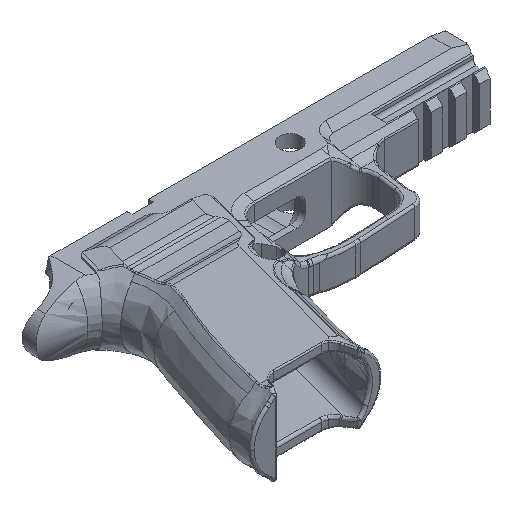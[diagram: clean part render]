
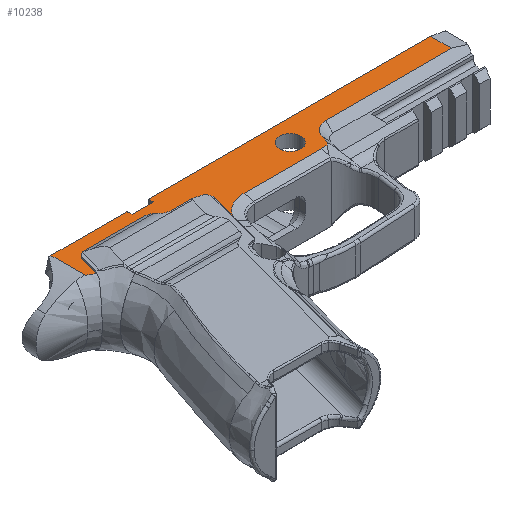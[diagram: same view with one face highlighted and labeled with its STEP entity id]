
A CAD part, isometric view. The second image highlights one B-rep face of the part: STEP entity #10238.
In plain terms, the highlighted planar face has unit normal (0, 0, 1).
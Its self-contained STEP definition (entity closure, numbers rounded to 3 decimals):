
#46=FACE_BOUND('',#2252,.T.);
#893=CIRCLE('',#10414,2.5);
#912=CIRCLE('',#10446,18.645);
#917=CIRCLE('',#10456,12.417);
#925=CIRCLE('',#10469,2.5);
#933=CIRCLE('',#10485,2.5);
#935=CIRCLE('',#10489,4.);
#1196=CIRCLE('',#11044,6.66);
#1201=CIRCLE('',#11060,4.45);
#1698=FACE_OUTER_BOUND('',#2251,.T.);
#2251=EDGE_LOOP('',(#8868,#8869,#8870,#8871,#8872,#8873,#8874,#8875,#8876,
#8877,#8878,#8879,#8880,#8881,#8882,#8883,#8884,#8885,#8886,#8887,#8888,
#8889,#8890));
#2252=EDGE_LOOP('',(#8891));
#2408=LINE('',#13754,#3114);
#2430=LINE('',#17517,#3136);
#2440=LINE('',#17562,#3146);
#2452=LINE('',#17637,#3158);
#2464=LINE('',#17746,#3170);
#2520=LINE('',#18097,#3226);
#2538=LINE('',#18163,#3244);
#2541=LINE('',#18167,#3247);
#2556=LINE('',#18329,#3262);
#2572=LINE('',#18667,#3278);
#2890=LINE('',#43894,#3596);
#2900=LINE('',#43918,#3606);
#2908=LINE('',#43935,#3614);
#2917=LINE('',#44001,#3623);
#2921=LINE('',#44007,#3627);
#2923=LINE('',#44013,#3629);
#3114=VECTOR('',#11300,10.);
#3136=VECTOR('',#11360,10.);
#3146=VECTOR('',#11382,10.);
#3158=VECTOR('',#11414,10.);
#3170=VECTOR('',#11458,10.);
#3226=VECTOR('',#11618,10.);
#3244=VECTOR('',#11670,10.);
#3247=VECTOR('',#11675,10.);
#3262=VECTOR('',#11728,10.);
#3278=VECTOR('',#11776,10.);
#3596=VECTOR('',#13082,10.);
#3606=VECTOR('',#13102,10.);
#3614=VECTOR('',#13118,10.);
#3623=VECTOR('',#13139,10.);
#3627=VECTOR('',#13145,10.);
#3629=VECTOR('',#13153,10.);
#3818=VERTEX_POINT('',#13751);
#3819=VERTEX_POINT('',#13753);
#3869=VERTEX_POINT('',#17515);
#3870=VERTEX_POINT('',#17516);
#3874=VERTEX_POINT('',#17526);
#3875=VERTEX_POINT('',#17527);
#3885=VERTEX_POINT('',#17554);
#3886=VERTEX_POINT('',#17561);
#3906=VERTEX_POINT('',#17634);
#3907=VERTEX_POINT('',#17636);
#3928=VERTEX_POINT('',#17739);
#3933=VERTEX_POINT('',#17835);
#3958=VERTEX_POINT('',#17917);
#3991=VERTEX_POINT('',#18045);
#3992=VERTEX_POINT('',#18046);
#4007=VERTEX_POINT('',#18094);
#4008=VERTEX_POINT('',#18096);
#4035=VERTEX_POINT('',#18162);
#4626=VERTEX_POINT('',#43891);
#4627=VERTEX_POINT('',#43893);
#4636=VERTEX_POINT('',#43917);
#4649=VERTEX_POINT('',#43998);
#4650=VERTEX_POINT('',#44000);
#4652=VERTEX_POINT('',#44009);
#4862=EDGE_CURVE('',#3819,#3818,#2408,.T.);
#4919=EDGE_CURVE('',#3869,#3870,#2430,.T.);
#4924=EDGE_CURVE('',#3874,#3875,#893,.T.);
#4935=EDGE_CURVE('',#3886,#3885,#2440,.T.);
#4957=EDGE_CURVE('',#3907,#3906,#2452,.T.);
#4983=EDGE_CURVE('',#3906,#3928,#2464,.T.);
#4988=EDGE_CURVE('',#3928,#3933,#912,.T.);
#5019=EDGE_CURVE('',#3885,#3958,#917,.T.);
#5036=EDGE_CURVE('',#3870,#3886,#925,.T.);
#5060=EDGE_CURVE('',#3991,#3992,#933,.T.);
#5066=EDGE_CURVE('',#3875,#3869,#935,.T.);
#5079=EDGE_CURVE('',#4008,#4007,#2520,.T.);
#5110=EDGE_CURVE('',#4035,#4008,#2538,.T.);
#5113=EDGE_CURVE('',#4007,#3907,#2541,.T.);
#5144=EDGE_CURVE('',#3933,#3991,#2556,.T.);
#5175=EDGE_CURVE('',#3992,#3874,#2572,.T.);
#6090=EDGE_CURVE('',#4626,#4627,#2890,.T.);
#6092=EDGE_CURVE('',#4626,#3819,#1196,.T.);
#6101=EDGE_CURVE('',#3818,#4636,#2900,.T.);
#6110=EDGE_CURVE('',#4636,#4035,#2908,.T.);
#6122=EDGE_CURVE('',#4649,#4650,#2917,.T.);
#6126=EDGE_CURVE('',#3958,#4650,#2921,.T.);
#6127=EDGE_CURVE('',#4652,#4652,#1201,.T.);
#6129=EDGE_CURVE('',#4649,#4627,#2923,.T.);
#8868=ORIENTED_EDGE('',*,*,#6110,.T.);
#8869=ORIENTED_EDGE('',*,*,#5110,.T.);
#8870=ORIENTED_EDGE('',*,*,#5079,.T.);
#8871=ORIENTED_EDGE('',*,*,#5113,.T.);
#8872=ORIENTED_EDGE('',*,*,#4957,.T.);
#8873=ORIENTED_EDGE('',*,*,#4983,.T.);
#8874=ORIENTED_EDGE('',*,*,#4988,.T.);
#8875=ORIENTED_EDGE('',*,*,#5144,.T.);
#8876=ORIENTED_EDGE('',*,*,#5060,.T.);
#8877=ORIENTED_EDGE('',*,*,#5175,.T.);
#8878=ORIENTED_EDGE('',*,*,#4924,.T.);
#8879=ORIENTED_EDGE('',*,*,#5066,.T.);
#8880=ORIENTED_EDGE('',*,*,#4919,.T.);
#8881=ORIENTED_EDGE('',*,*,#5036,.T.);
#8882=ORIENTED_EDGE('',*,*,#4935,.T.);
#8883=ORIENTED_EDGE('',*,*,#5019,.T.);
#8884=ORIENTED_EDGE('',*,*,#6126,.T.);
#8885=ORIENTED_EDGE('',*,*,#6122,.F.);
#8886=ORIENTED_EDGE('',*,*,#6129,.T.);
#8887=ORIENTED_EDGE('',*,*,#6090,.F.);
#8888=ORIENTED_EDGE('',*,*,#6092,.T.);
#8889=ORIENTED_EDGE('',*,*,#4862,.T.);
#8890=ORIENTED_EDGE('',*,*,#6101,.T.);
#8891=ORIENTED_EDGE('',*,*,#6127,.T.);
#9747=PLANE('',#11061);
#10238=ADVANCED_FACE('',(#1698,#46),#9747,.T.);
#10414=AXIS2_PLACEMENT_3D('',#17528,#11368,#11369);
#10446=AXIS2_PLACEMENT_3D('',#17842,#11464,#11465);
#10456=AXIS2_PLACEMENT_3D('',#17919,#11509,#11510);
#10469=AXIS2_PLACEMENT_3D('',#17955,#11544,#11545);
#10485=AXIS2_PLACEMENT_3D('',#18047,#11587,#11588);
#10489=AXIS2_PLACEMENT_3D('',#18061,#11597,#11598);
#11044=AXIS2_PLACEMENT_3D('',#43897,#13086,#13087);
#11060=AXIS2_PLACEMENT_3D('',#44010,#13148,#13149);
#11061=AXIS2_PLACEMENT_3D('',#44012,#13151,#13152);
#11300=DIRECTION('',(1.,0.,0.));
#11360=DIRECTION('',(1.,0.,0.));
#11368=DIRECTION('center_axis',(0.,0.,-1.));
#11369=DIRECTION('ref_axis',(0.973,0.231,0.));
#11382=DIRECTION('',(-0.259,-0.966,0.));
#11414=DIRECTION('',(-1.,0.,0.));
#11458=DIRECTION('',(0.,-1.,0.));
#11464=DIRECTION('center_axis',(0.,0.,-1.));
#11465=DIRECTION('ref_axis',(0.608,0.794,0.));
#11509=DIRECTION('center_axis',(0.,0.,-1.));
#11510=DIRECTION('ref_axis',(-0.939,0.345,0.));
#11544=DIRECTION('center_axis',(0.,0.,-1.));
#11545=DIRECTION('ref_axis',(0.966,-0.259,0.));
#11587=DIRECTION('center_axis',(0.,0.,-1.));
#11588=DIRECTION('ref_axis',(0.,1.,0.));
#11597=DIRECTION('center_axis',(0.,0.,1.));
#11598=DIRECTION('ref_axis',(-0.973,-0.231,0.));
#11618=DIRECTION('',(-1.,0.,0.));
#11670=DIRECTION('',(0.,-1.,0.));
#11675=DIRECTION('',(0.,1.,0.));
#11728=DIRECTION('',(0.259,0.966,0.));
#11776=DIRECTION('',(1.,0.,0.));
#13082=DIRECTION('',(-0.259,-0.966,0.));
#13086=DIRECTION('center_axis',(0.,0.,-1.));
#13087=DIRECTION('ref_axis',(0.,1.,0.));
#13102=DIRECTION('',(0.,1.,0.));
#13118=DIRECTION('',(-1.,0.,0.));
#13139=DIRECTION('',(-1.,0.,0.));
#13145=DIRECTION('',(1.,0.,0.));
#13148=DIRECTION('center_axis',(0.,0.,-1.));
#13149=DIRECTION('ref_axis',(1.,0.,0.));
#13151=DIRECTION('center_axis',(0.,0.,1.));
#13152=DIRECTION('ref_axis',(1.,0.,0.));
#13153=DIRECTION('',(0.793,0.609,0.));
#13751=CARTESIAN_POINT('',(66.9,0.46,13.5));
#13753=CARTESIAN_POINT('',(15.11,0.46,13.5));
#13754=CARTESIAN_POINT('',(26.85,0.46,13.5));
#17515=CARTESIAN_POINT('',(-50.999,-2.,13.5));
#17516=CARTESIAN_POINT('',(-38.372,-2.,13.5));
#17517=CARTESIAN_POINT('',(-35.15,-2.,13.5));
#17526=CARTESIAN_POINT('',(-57.324,3.,13.5));
#17527=CARTESIAN_POINT('',(-54.891,1.077,13.5));
#17528=CARTESIAN_POINT('Origin',(-57.324,0.5,13.5));
#17554=CARTESIAN_POINT('',(-38.684,-15.324,13.5));
#17561=CARTESIAN_POINT('',(-35.957,-5.147,13.5));
#17562=CARTESIAN_POINT('',(-40.35,-21.54,13.5));
#17634=CARTESIAN_POINT('',(-89.671,9.,13.5));
#17636=CARTESIAN_POINT('',(-58.2,9.,13.5));
#17637=CARTESIAN_POINT('',(-111.6,9.,13.5));
#17739=CARTESIAN_POINT('',(-89.671,-5.18,13.5));
#17746=CARTESIAN_POINT('',(-89.671,9.,13.5));
#17835=CARTESIAN_POINT('',(-86.745,-6.914,13.5));
#17842=CARTESIAN_POINT('Origin',(-97.678,-22.018,13.5));
#17917=CARTESIAN_POINT('',(-27.64,-8.583,13.5));
#17919=CARTESIAN_POINT('Origin',(-27.64,-21.,13.5));
#17955=CARTESIAN_POINT('Origin',(-38.372,-4.5,13.5));
#18045=CARTESIAN_POINT('',(-84.585,1.147,13.5));
#18046=CARTESIAN_POINT('',(-82.17,3.,13.5));
#18047=CARTESIAN_POINT('Origin',(-82.17,0.5,13.5));
#18061=CARTESIAN_POINT('Origin',(-50.999,2.,13.5));
#18094=CARTESIAN_POINT('',(-58.2,7.,13.5));
#18096=CARTESIAN_POINT('',(-49.5,7.,13.5));
#18097=CARTESIAN_POINT('',(-38.75,7.,13.5));
#18162=CARTESIAN_POINT('',(-49.5,9.,13.5));
#18163=CARTESIAN_POINT('',(-49.5,-18.875,13.5));
#18167=CARTESIAN_POINT('',(-58.2,-17.875,13.5));
#18329=CARTESIAN_POINT('',(-90.32,-20.255,13.5));
#18667=CARTESIAN_POINT('',(-50.735,3.,13.5));
#43891=CARTESIAN_POINT('',(8.677,-4.476,13.5));
#43893=CARTESIAN_POINT('',(7.816,-7.69,13.5));
#43894=CARTESIAN_POINT('',(2.706,-26.761,13.5));
#43897=CARTESIAN_POINT('Origin',(15.11,-6.2,13.5));
#43917=CARTESIAN_POINT('',(66.9,9.,13.5));
#43918=CARTESIAN_POINT('',(66.9,-17.875,13.5));
#43935=CARTESIAN_POINT('',(-111.6,9.,13.5));
#43998=CARTESIAN_POINT('',(6.653,-8.583,13.5));
#44000=CARTESIAN_POINT('',(4.179,-8.583,13.5));
#44001=CARTESIAN_POINT('',(4.179,-8.583,13.5));
#44007=CARTESIAN_POINT('',(-15.515,-8.583,13.5));
#44009=CARTESIAN_POINT('',(-4.45,0.,13.5));
#44010=CARTESIAN_POINT('Origin',(0.,0.,13.5));
#44012=CARTESIAN_POINT('Origin',(-19.3,-44.75,13.5));
#44013=CARTESIAN_POINT('',(-9.667,-21.105,13.5));
